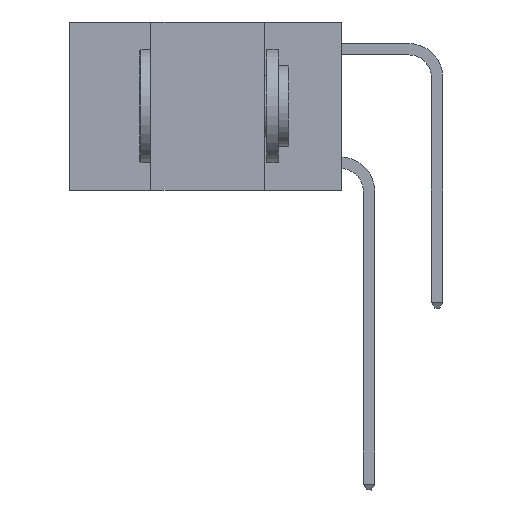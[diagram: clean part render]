
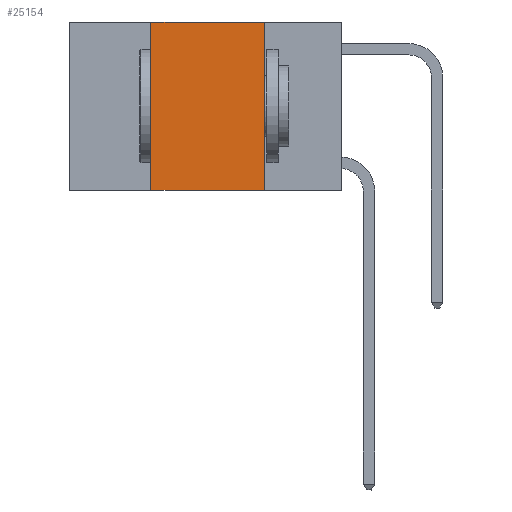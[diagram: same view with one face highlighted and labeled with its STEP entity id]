
A CAD part, left-side view. The second image highlights one B-rep face of the part: STEP entity #25154.
In plain terms, the highlighted planar face has unit normal (-1, 0, 0).
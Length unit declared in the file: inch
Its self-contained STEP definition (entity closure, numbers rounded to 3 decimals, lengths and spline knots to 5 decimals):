
#328 = VECTOR ( 'NONE', #2285, 39.37008 ) ;
#596 = EDGE_CURVE ( 'NONE', #6116, #16898, #4248, .T. ) ;
#1505 = EDGE_CURVE ( 'NONE', #6116, #7195, #13556, .T. ) ;
#2285 = DIRECTION ( 'NONE',  ( 0., -1., 0. ) ) ;
#2668 = DIRECTION ( 'NONE',  ( 1., 0., 0. ) ) ;
#3245 = ORIENTED_EDGE ( 'NONE', *, *, #596, .T. ) ;
#4248 = LINE ( 'NONE', #20106, #328 ) ;
#4528 = DIRECTION ( 'NONE',  ( 0., -1., 0. ) ) ;
#5730 = CARTESIAN_POINT ( 'NONE',  ( 0., 0.17, -0.37 ) ) ;
#6116 = VERTEX_POINT ( 'NONE', #15631 ) ;
#6291 = EDGE_CURVE ( 'NONE', #21053, #16898, #6476, .T. ) ;
#6316 = CARTESIAN_POINT ( 'NONE',  ( 0., 0.6, 0. ) ) ;
#6476 = LINE ( 'NONE', #19882, #9378 ) ;
#7195 = VERTEX_POINT ( 'NONE', #17771 ) ;
#8040 = DIRECTION ( 'NONE',  ( 0., 0., -1. ) ) ;
#9378 = VECTOR ( 'NONE', #8040, 39.37008 ) ;
#10181 = CARTESIAN_POINT ( 'NONE',  ( 0., 0.42, 0. ) ) ;
#10220 = ORIENTED_EDGE ( 'NONE', *, *, #22062, .F. ) ;
#10614 = DIRECTION ( 'NONE',  ( 0., 0., -1. ) ) ;
#12168 = PLANE ( 'NONE',  #20493 ) ;
#12301 = FACE_OUTER_BOUND ( 'NONE', #24911, .T. ) ;
#13556 = LINE ( 'NONE', #10181, #14912 ) ;
#14152 = LINE ( 'NONE', #20125, #24201 ) ;
#14912 = VECTOR ( 'NONE', #25709, 39.37008 ) ;
#15631 = CARTESIAN_POINT ( 'NONE',  ( 0., 0.42, -0.37 ) ) ;
#16898 = VERTEX_POINT ( 'NONE', #5730 ) ;
#17771 = CARTESIAN_POINT ( 'NONE',  ( 0., 0.42, 0. ) ) ;
#17793 = ORIENTED_EDGE ( 'NONE', *, *, #1505, .F. ) ;
#19882 = CARTESIAN_POINT ( 'NONE',  ( 0., 0.17, 0. ) ) ;
#20106 = CARTESIAN_POINT ( 'NONE',  ( 0., 0.6, -0.37 ) ) ;
#20125 = CARTESIAN_POINT ( 'NONE',  ( 0., 0.6, 0. ) ) ;
#20493 = AXIS2_PLACEMENT_3D ( 'NONE', #6316, #2668, #10614 ) ;
#21053 = VERTEX_POINT ( 'NONE', #23791 ) ;
#22062 = EDGE_CURVE ( 'NONE', #7195, #21053, #14152, .T. ) ;
#23303 = ORIENTED_EDGE ( 'NONE', *, *, #6291, .F. ) ;
#23791 = CARTESIAN_POINT ( 'NONE',  ( 0., 0.17, 0. ) ) ;
#24201 = VECTOR ( 'NONE', #4528, 39.37008 ) ;
#24911 = EDGE_LOOP ( 'NONE', ( #23303, #10220, #17793, #3245 ) ) ;
#25154 = ADVANCED_FACE ( 'NONE', ( #12301 ), #12168, .F. ) ;
#25709 = DIRECTION ( 'NONE',  ( 0., 0., 1. ) ) ;
